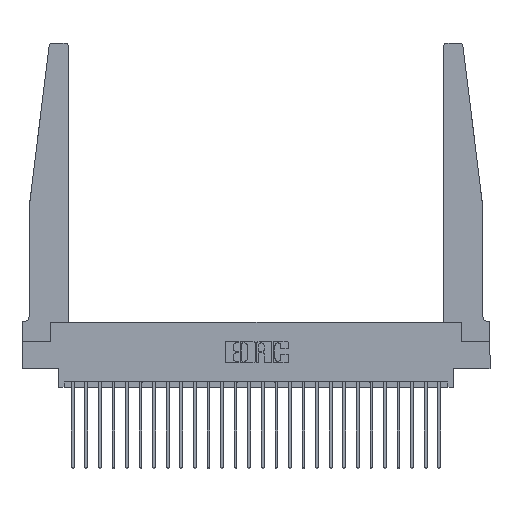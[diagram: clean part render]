
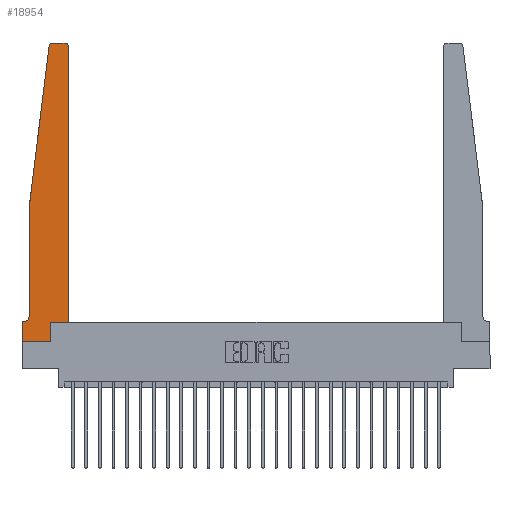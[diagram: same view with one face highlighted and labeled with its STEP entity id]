
A CAD part, top view. The second image highlights one B-rep face of the part: STEP entity #18954.
In plain terms, the highlighted planar face has unit normal (0, 0, 1).
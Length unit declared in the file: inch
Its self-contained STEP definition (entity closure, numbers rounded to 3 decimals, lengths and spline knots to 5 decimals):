
#1 = CARTESIAN_POINT ( 'NONE',  ( 0.065, 1.25, 0.37 ) ) ;
#136 = ORIENTED_EDGE ( 'NONE', *, *, #8754, .T. ) ;
#199 = EDGE_CURVE ( 'NONE', #6260, #10138, #23357, .T. ) ;
#232 = DIRECTION ( 'NONE',  ( -1., 0., 0. ) ) ;
#246 = DIRECTION ( 'NONE',  ( 0., 1., 0. ) ) ;
#537 = AXIS2_PLACEMENT_3D ( 'NONE', #14726, #3007, #16645 ) ;
#679 = VERTEX_POINT ( 'NONE', #20631 ) ;
#772 = VECTOR ( 'NONE', #6189, 39.37008 ) ;
#976 = ORIENTED_EDGE ( 'NONE', *, *, #23195, .T. ) ;
#1303 = AXIS2_PLACEMENT_3D ( 'NONE', #7646, #9571, #22977 ) ;
#1644 = CARTESIAN_POINT ( 'NONE',  ( 0.065, 1.25, 0.37 ) ) ;
#1648 = CARTESIAN_POINT ( 'NONE',  ( 0.015, 0.1875, 0.37 ) ) ;
#1956 = LINE ( 'NONE', #1, #21977 ) ;
#1990 = DIRECTION ( 'NONE',  ( 0., -1., 0. ) ) ;
#2001 = ORIENTED_EDGE ( 'NONE', *, *, #5234, .T. ) ;
#2301 = LINE ( 'NONE', #19416, #22285 ) ;
#3007 = DIRECTION ( 'NONE',  ( 0., 0., 1. ) ) ;
#3062 = VERTEX_POINT ( 'NONE', #21469 ) ;
#3399 = VERTEX_POINT ( 'NONE', #13362 ) ;
#3672 = DIRECTION ( 'NONE',  ( -0.122, -0.992, 0. ) ) ;
#3796 = VERTEX_POINT ( 'NONE', #6591 ) ;
#4016 = CARTESIAN_POINT ( 'NONE',  ( 0.015, 0.2375, 0.37 ) ) ;
#4144 = CARTESIAN_POINT ( 'NONE',  ( 0.425, 0.18, 0.37 ) ) ;
#4419 = ORIENTED_EDGE ( 'NONE', *, *, #16223, .T. ) ;
#4939 = CIRCLE ( 'NONE', #537, 0.03 ) ;
#4990 = CARTESIAN_POINT ( 'NONE',  ( 0.27653, 2.75, 0.37 ) ) ;
#5067 = AXIS2_PLACEMENT_3D ( 'NONE', #16932, #5314, #18832 ) ;
#5234 = EDGE_CURVE ( 'NONE', #679, #3796, #1956, .T. ) ;
#5314 = DIRECTION ( 'NONE',  ( 0., 0., 1. ) ) ;
#5381 = CIRCLE ( 'NONE', #5067, 0.03 ) ;
#5660 = PLANE ( 'NONE',  #1303 ) ;
#5731 = VECTOR ( 'NONE', #246, 39.37008 ) ;
#5848 = EDGE_CURVE ( 'NONE', #10473, #19940, #19901, .T. ) ;
#6036 = DIRECTION ( 'NONE',  ( -1., 0., 0. ) ) ;
#6189 = DIRECTION ( 'NONE',  ( 0., 1., 0. ) ) ;
#6260 = VERTEX_POINT ( 'NONE', #15061 ) ;
#6393 = VECTOR ( 'NONE', #14968, 39.37008 ) ;
#6591 = CARTESIAN_POINT ( 'NONE',  ( 0.065, 0.2375, 0.37 ) ) ;
#6728 = CARTESIAN_POINT ( 'NONE',  ( 0.065, 0.1875, 0.37 ) ) ;
#7023 = EDGE_CURVE ( 'NONE', #3796, #22357, #22516, .T. ) ;
#7055 = VERTEX_POINT ( 'NONE', #21413 ) ;
#7393 = CARTESIAN_POINT ( 'NONE',  ( 0.24675, 2.72367, 0.37 ) ) ;
#7592 = LINE ( 'NONE', #22508, #6393 ) ;
#7646 = CARTESIAN_POINT ( 'NONE',  ( 0., 0.1875, 0.37 ) ) ;
#7854 = EDGE_LOOP ( 'NONE', ( #20737, #20281, #8377, #2001, #22680, #136, #20964, #21306, #21828, #4419, #21514, #976 ) ) ;
#8377 = ORIENTED_EDGE ( 'NONE', *, *, #24671, .T. ) ;
#8754 = EDGE_CURVE ( 'NONE', #22357, #7055, #9262, .T. ) ;
#9262 = LINE ( 'NONE', #6728, #20077 ) ;
#9377 = LINE ( 'NONE', #9872, #14280 ) ;
#9411 = EDGE_CURVE ( 'NONE', #10138, #23235, #4939, .T. ) ;
#9571 = DIRECTION ( 'NONE',  ( 0., 0., 1. ) ) ;
#9872 = CARTESIAN_POINT ( 'NONE',  ( 0., 0., 0.37 ) ) ;
#10138 = VERTEX_POINT ( 'NONE', #4990 ) ;
#10195 = AXIS2_PLACEMENT_3D ( 'NONE', #4016, #17609, #6036 ) ;
#10260 = CARTESIAN_POINT ( 'NONE',  ( 0.2605, 0., 0.37 ) ) ;
#10473 = VERTEX_POINT ( 'NONE', #10260 ) ;
#12020 = CARTESIAN_POINT ( 'NONE',  ( 0.2605, 0.18, 0.37 ) ) ;
#12577 = EDGE_CURVE ( 'NONE', #13213, #3062, #20810, .T. ) ;
#13213 = VERTEX_POINT ( 'NONE', #22586 ) ;
#13362 = CARTESIAN_POINT ( 'NONE',  ( 0., 0., 0.37 ) ) ;
#13741 = CARTESIAN_POINT ( 'NONE',  ( 0.25, 2.75, 0.37 ) ) ;
#13759 = DIRECTION ( 'NONE',  ( 1., 0., 0. ) ) ;
#13816 = FACE_OUTER_BOUND ( 'NONE', #7854, .T. ) ;
#14280 = VECTOR ( 'NONE', #15740, 39.37008 ) ;
#14726 = CARTESIAN_POINT ( 'NONE',  ( 0.27653, 2.72, 0.37 ) ) ;
#14968 = DIRECTION ( 'NONE',  ( 1., 0., 0. ) ) ;
#15061 = CARTESIAN_POINT ( 'NONE',  ( 0.395, 2.75, 0.37 ) ) ;
#15564 = CARTESIAN_POINT ( 'NONE',  ( 0.2605, 0.18, 0.37 ) ) ;
#15740 = DIRECTION ( 'NONE',  ( 0., -1., 0. ) ) ;
#15819 = EDGE_CURVE ( 'NONE', #7055, #3399, #9377, .T. ) ;
#16223 = EDGE_CURVE ( 'NONE', #19940, #13213, #7592, .T. ) ;
#16645 = DIRECTION ( 'NONE',  ( 1., 0., 0. ) ) ;
#16932 = CARTESIAN_POINT ( 'NONE',  ( 0.395, 2.72, 0.37 ) ) ;
#17609 = DIRECTION ( 'NONE',  ( 0., 0., -1. ) ) ;
#18265 = DIRECTION ( 'NONE',  ( -1., 0., 0. ) ) ;
#18832 = DIRECTION ( 'NONE',  ( 1., 0., 0. ) ) ;
#18891 = VECTOR ( 'NONE', #232, 39.37008 ) ;
#18954 = ADVANCED_FACE ( 'NONE', ( #13816 ), #5660, .T. ) ;
#19416 = CARTESIAN_POINT ( 'NONE',  ( 0., 0., 0.37 ) ) ;
#19837 = LINE ( 'NONE', #1644, #23701 ) ;
#19901 = LINE ( 'NONE', #12020, #5731 ) ;
#19940 = VERTEX_POINT ( 'NONE', #15564 ) ;
#20077 = VECTOR ( 'NONE', #18265, 39.37008 ) ;
#20281 = ORIENTED_EDGE ( 'NONE', *, *, #9411, .T. ) ;
#20631 = CARTESIAN_POINT ( 'NONE',  ( 0.065, 1.25, 0.37 ) ) ;
#20737 = ORIENTED_EDGE ( 'NONE', *, *, #199, .T. ) ;
#20810 = LINE ( 'NONE', #4144, #772 ) ;
#20964 = ORIENTED_EDGE ( 'NONE', *, *, #15819, .T. ) ;
#21306 = ORIENTED_EDGE ( 'NONE', *, *, #22443, .T. ) ;
#21413 = CARTESIAN_POINT ( 'NONE',  ( 0., 0.1875, 0.37 ) ) ;
#21469 = CARTESIAN_POINT ( 'NONE',  ( 0.425, 2.72, 0.37 ) ) ;
#21514 = ORIENTED_EDGE ( 'NONE', *, *, #12577, .T. ) ;
#21828 = ORIENTED_EDGE ( 'NONE', *, *, #5848, .T. ) ;
#21977 = VECTOR ( 'NONE', #1990, 39.37008 ) ;
#22285 = VECTOR ( 'NONE', #13759, 39.37008 ) ;
#22357 = VERTEX_POINT ( 'NONE', #1648 ) ;
#22443 = EDGE_CURVE ( 'NONE', #3399, #10473, #2301, .T. ) ;
#22508 = CARTESIAN_POINT ( 'NONE',  ( 0.425, 0.18, 0.37 ) ) ;
#22516 = CIRCLE ( 'NONE', #10195, 0.05 ) ;
#22586 = CARTESIAN_POINT ( 'NONE',  ( 0.425, 0.18, 0.37 ) ) ;
#22680 = ORIENTED_EDGE ( 'NONE', *, *, #7023, .T. ) ;
#22977 = DIRECTION ( 'NONE',  ( 1., 0., 0. ) ) ;
#23195 = EDGE_CURVE ( 'NONE', #3062, #6260, #5381, .T. ) ;
#23235 = VERTEX_POINT ( 'NONE', #7393 ) ;
#23357 = LINE ( 'NONE', #13741, #18891 ) ;
#23701 = VECTOR ( 'NONE', #3672, 39.37008 ) ;
#24671 = EDGE_CURVE ( 'NONE', #23235, #679, #19837, .T. ) ;
